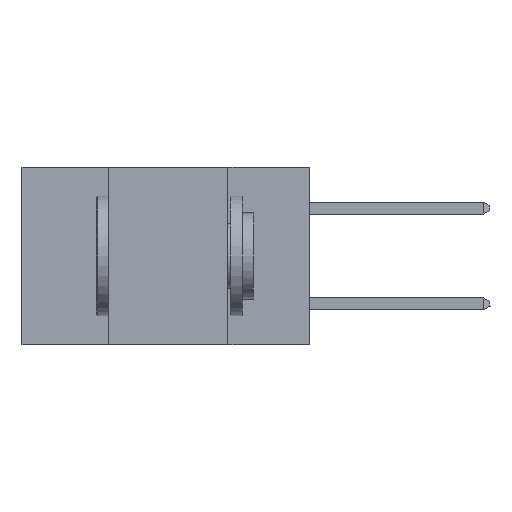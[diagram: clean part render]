
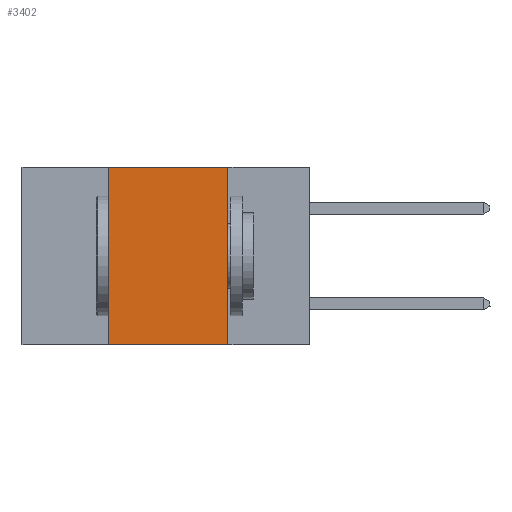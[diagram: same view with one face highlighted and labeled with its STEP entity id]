
A CAD part, left-side view. The second image highlights one B-rep face of the part: STEP entity #3402.
In plain terms, the highlighted planar face has unit normal (-1, 0, 0).
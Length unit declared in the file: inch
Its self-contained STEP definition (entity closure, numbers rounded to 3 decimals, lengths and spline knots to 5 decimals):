
#27 = FACE_OUTER_BOUND ( 'NONE', #3713, .T. ) ;
#183 = VECTOR ( 'NONE', #5215, 39.37008 ) ;
#422 = CARTESIAN_POINT ( 'NONE',  ( 0., 0.17, -0.37 ) ) ;
#772 = ORIENTED_EDGE ( 'NONE', *, *, #7582, .F. ) ;
#902 = VECTOR ( 'NONE', #9398, 39.37008 ) ;
#1278 = CARTESIAN_POINT ( 'NONE',  ( 0., 0.42, -0.37 ) ) ;
#1498 = EDGE_CURVE ( 'NONE', #6411, #5595, #6187, .T. ) ;
#1627 = CARTESIAN_POINT ( 'NONE',  ( 0., 0.17, 0. ) ) ;
#1675 = CARTESIAN_POINT ( 'NONE',  ( 0., 0.42, 0. ) ) ;
#1689 = VERTEX_POINT ( 'NONE', #1627 ) ;
#2181 = LINE ( 'NONE', #3716, #9600 ) ;
#2972 = LINE ( 'NONE', #4326, #902 ) ;
#3054 = CARTESIAN_POINT ( 'NONE',  ( 0., 0.42, 0. ) ) ;
#3074 = ORIENTED_EDGE ( 'NONE', *, *, #1498, .F. ) ;
#3402 = ADVANCED_FACE ( 'NONE', ( #27 ), #9389, .F. ) ;
#3713 = EDGE_LOOP ( 'NONE', ( #7939, #772, #3074, #7409 ) ) ;
#3716 = CARTESIAN_POINT ( 'NONE',  ( 0., 0.17, 0. ) ) ;
#4156 = AXIS2_PLACEMENT_3D ( 'NONE', #9139, #9355, #9647 ) ;
#4326 = CARTESIAN_POINT ( 'NONE',  ( 0., 0.6, -0.37 ) ) ;
#4443 = CARTESIAN_POINT ( 'NONE',  ( 0., 0.6, 0. ) ) ;
#4643 = EDGE_CURVE ( 'NONE', #1689, #5889, #2181, .T. ) ;
#5215 = DIRECTION ( 'NONE',  ( 0., 0., 1. ) ) ;
#5241 = DIRECTION ( 'NONE',  ( 0., -1., 0. ) ) ;
#5595 = VERTEX_POINT ( 'NONE', #1675 ) ;
#5807 = DIRECTION ( 'NONE',  ( 0., 0., -1. ) ) ;
#5889 = VERTEX_POINT ( 'NONE', #422 ) ;
#5929 = VECTOR ( 'NONE', #5241, 39.37008 ) ;
#6149 = LINE ( 'NONE', #4443, #5929 ) ;
#6187 = LINE ( 'NONE', #3054, #183 ) ;
#6411 = VERTEX_POINT ( 'NONE', #1278 ) ;
#7409 = ORIENTED_EDGE ( 'NONE', *, *, #8107, .T. ) ;
#7582 = EDGE_CURVE ( 'NONE', #5595, #1689, #6149, .T. ) ;
#7939 = ORIENTED_EDGE ( 'NONE', *, *, #4643, .F. ) ;
#8107 = EDGE_CURVE ( 'NONE', #6411, #5889, #2972, .T. ) ;
#9139 = CARTESIAN_POINT ( 'NONE',  ( 0., 0.6, 0. ) ) ;
#9355 = DIRECTION ( 'NONE',  ( 1., 0., 0. ) ) ;
#9389 = PLANE ( 'NONE',  #4156 ) ;
#9398 = DIRECTION ( 'NONE',  ( 0., -1., 0. ) ) ;
#9600 = VECTOR ( 'NONE', #5807, 39.37008 ) ;
#9647 = DIRECTION ( 'NONE',  ( 0., 0., -1. ) ) ;
